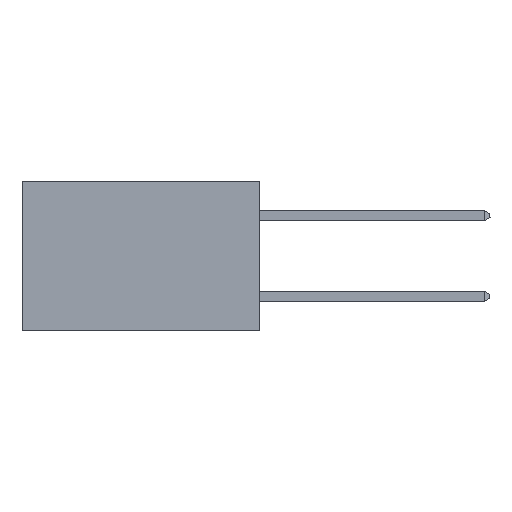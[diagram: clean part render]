
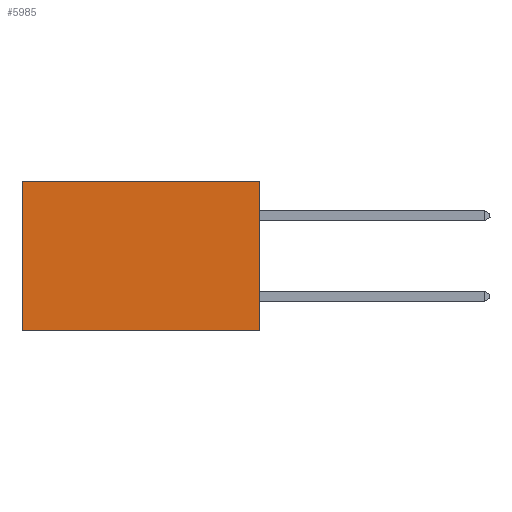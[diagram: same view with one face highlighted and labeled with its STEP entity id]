
A CAD part, left-side view. The second image highlights one B-rep face of the part: STEP entity #5985.
In plain terms, the highlighted planar face has unit normal (-1, 0, 0).
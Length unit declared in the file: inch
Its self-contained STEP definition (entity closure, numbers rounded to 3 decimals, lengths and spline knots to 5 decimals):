
#195 = CARTESIAN_POINT ( 'NONE',  ( 0.277, 0.59, 0. ) ) ;
#1238 = ORIENTED_EDGE ( 'NONE', *, *, #7627, .F. ) ;
#1434 = ORIENTED_EDGE ( 'NONE', *, *, #30856, .T. ) ;
#1749 = FACE_OUTER_BOUND ( 'NONE', #26273, .T. ) ;
#3363 = VERTEX_POINT ( 'NONE', #14366 ) ;
#3481 = LINE ( 'NONE', #6758, #28543 ) ;
#4831 = ORIENTED_EDGE ( 'NONE', *, *, #22095, .F. ) ;
#5985 = ADVANCED_FACE ( 'NONE', ( #1749 ), #18815, .F. ) ;
#6758 = CARTESIAN_POINT ( 'NONE',  ( 0.277, 0., -0.37 ) ) ;
#7490 = VECTOR ( 'NONE', #9862, 39.37008 ) ;
#7627 = EDGE_CURVE ( 'NONE', #26219, #8614, #29461, .T. ) ;
#7890 = DIRECTION ( 'NONE',  ( 0., 0., -1. ) ) ;
#8614 = VERTEX_POINT ( 'NONE', #24794 ) ;
#9161 = VECTOR ( 'NONE', #7890, 39.37008 ) ;
#9862 = DIRECTION ( 'NONE',  ( 0., 1., 0. ) ) ;
#13570 = ORIENTED_EDGE ( 'NONE', *, *, #21595, .T. ) ;
#14100 = LINE ( 'NONE', #19671, #7490 ) ;
#14366 = CARTESIAN_POINT ( 'NONE',  ( 0.277, 0.59, -0.37 ) ) ;
#17372 = AXIS2_PLACEMENT_3D ( 'NONE', #18950, #19462, #18741 ) ;
#18741 = DIRECTION ( 'NONE',  ( 0., 0., -1. ) ) ;
#18815 = PLANE ( 'NONE',  #17372 ) ;
#18950 = CARTESIAN_POINT ( 'NONE',  ( 0.277, 0., -0.37 ) ) ;
#19462 = DIRECTION ( 'NONE',  ( 1., 0., 0. ) ) ;
#19671 = CARTESIAN_POINT ( 'NONE',  ( 0.277, 0., 0. ) ) ;
#21595 = EDGE_CURVE ( 'NONE', #26219, #21705, #14100, .T. ) ;
#21705 = VERTEX_POINT ( 'NONE', #195 ) ;
#22095 = EDGE_CURVE ( 'NONE', #8614, #3363, #3481, .T. ) ;
#22477 = LINE ( 'NONE', #25393, #9161 ) ;
#22910 = VECTOR ( 'NONE', #23331, 39.37008 ) ;
#23331 = DIRECTION ( 'NONE',  ( 0., 0., -1. ) ) ;
#24794 = CARTESIAN_POINT ( 'NONE',  ( 0.277, 0., -0.37 ) ) ;
#25393 = CARTESIAN_POINT ( 'NONE',  ( 0.277, 0.59, -0.37 ) ) ;
#25913 = CARTESIAN_POINT ( 'NONE',  ( 0.277, 0., 0. ) ) ;
#26219 = VERTEX_POINT ( 'NONE', #25913 ) ;
#26273 = EDGE_LOOP ( 'NONE', ( #1434, #4831, #1238, #13570 ) ) ;
#28543 = VECTOR ( 'NONE', #31608, 39.37008 ) ;
#29461 = LINE ( 'NONE', #30731, #22910 ) ;
#30731 = CARTESIAN_POINT ( 'NONE',  ( 0.277, 0., -0.37 ) ) ;
#30856 = EDGE_CURVE ( 'NONE', #21705, #3363, #22477, .T. ) ;
#31608 = DIRECTION ( 'NONE',  ( 0., 1., 0. ) ) ;
